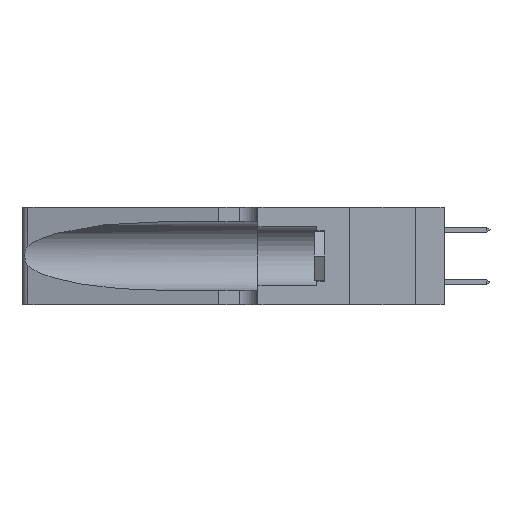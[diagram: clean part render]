
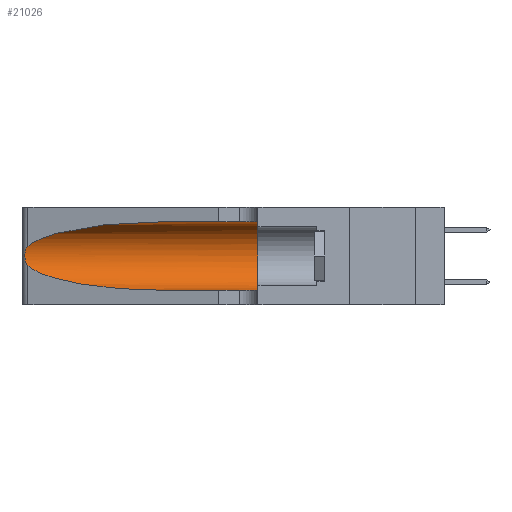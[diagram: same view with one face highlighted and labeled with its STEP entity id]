
A CAD part, left-side view. The second image highlights one B-rep face of the part: STEP entity #21026.
In plain terms, the highlighted cylindrical face has radius 3.308 mm (diameter 6.617 mm), a partial arc.
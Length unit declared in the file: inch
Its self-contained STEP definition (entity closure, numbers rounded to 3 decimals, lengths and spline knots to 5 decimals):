
#993 = CYLINDRICAL_SURFACE ( 'NONE', #23673, 0.13025 ) ;
#1187 = ORIENTED_EDGE ( 'NONE', *, *, #15606, .T. ) ;
#1344 = EDGE_CURVE ( 'NONE', #5291, #2969, #7598, .T. ) ;
#1790 = CARTESIAN_POINT ( 'NONE',  ( 0.1305, 0.35, 0.31525 ) ) ;
#2310 = CARTESIAN_POINT ( 'NONE',  ( 0.25555, 1.22993, 0.14849 ) ) ;
#2969 = VERTEX_POINT ( 'NONE', #16000 ) ;
#3154 = ORIENTED_EDGE ( 'NONE', *, *, #1344, .T. ) ;
#3229 = DIRECTION ( 'NONE',  ( 0., 0., -1. ) ) ;
#3460 = AXIS2_PLACEMENT_3D ( 'NONE', #23264, #11478, #3803 ) ;
#3540 = VERTEX_POINT ( 'NONE', #1790 ) ;
#3803 = DIRECTION ( 'NONE',  ( 0., 0., 1. ) ) ;
#4047 = VERTEX_POINT ( 'NONE', #6953 ) ;
#4234 = CARTESIAN_POINT ( 'NONE',  ( 0.25487, 1.22718, 0.22369 ) ) ;
#4408 = CARTESIAN_POINT ( 'NONE',  ( 0.26017, 1.23833, 0.17102 ) ) ;
#4570 = CARTESIAN_POINT ( 'NONE',  ( 0.1305, 1.61858, 0.05475 ) ) ;
#5130 = VECTOR ( 'NONE', #18428, 39.37008 ) ;
#5291 = VERTEX_POINT ( 'NONE', #11440 ) ;
#6953 = CARTESIAN_POINT ( 'NONE',  ( 0.1305, 0.72297, 0.31525 ) ) ;
#7598 = B_SPLINE_CURVE_WITH_KNOTS ( 'NONE', 3,
 ( #4234, #14229, #23850, #16210, #21959, #12078, #18184, #8489, #4408, #24016, #8404, #12253, #2310, #18264 ),
 .UNSPECIFIED., .F., .F.,
 ( 4, 2, 2, 2, 2, 2, 4 ),
 ( 0., 0.00027, 0.00053, 0.00107, 0.0016, 0.00187, 0.00214 ),
 .UNSPECIFIED. ) ;
#7819 = ORIENTED_EDGE ( 'NONE', *, *, #8131, .F. ) ;
#8131 = EDGE_CURVE ( 'NONE', #4047, #3540, #8203, .T. ) ;
#8194 = EDGE_CURVE ( 'NONE', #2969, #15204, #14914, .T. ) ;
#8203 = LINE ( 'NONE', #20918, #20862 ) ;
#8404 = CARTESIAN_POINT ( 'NONE',  ( 0.25789, 1.23486, 0.15765 ) ) ;
#8489 = CARTESIAN_POINT ( 'NONE',  ( 0.26075, 1.23896, 0.178 ) ) ;
#9005 = DIRECTION ( 'NONE',  ( 0., -1., 0. ) ) ;
#10164 = CARTESIAN_POINT ( 'NONE',  ( 0.25487, 1.22718, 0.14631 ) ) ;
#10472 =( BOUNDED_CURVE ( )  B_SPLINE_CURVE ( 3, ( #18890, #16655, #25178, #21300 ),
 .UNSPECIFIED., .F., .F. ) 
 B_SPLINE_CURVE_WITH_KNOTS ( ( 4, 4 ),
 ( 1.5708, 2.84003 ),
 .UNSPECIFIED. ) 
 CURVE ( )  GEOMETRIC_REPRESENTATION_ITEM ( )  RATIONAL_B_SPLINE_CURVE ( ( 1., 0.87, 0.87, 1. ) ) 
 REPRESENTATION_ITEM ( '' )  );
#11344 = CARTESIAN_POINT ( 'NONE',  ( 0.1305, 0.72297, 0.05475 ) ) ;
#11440 = CARTESIAN_POINT ( 'NONE',  ( 0.25487, 1.22718, 0.22369 ) ) ;
#11478 = DIRECTION ( 'NONE',  ( 0., 1., 0. ) ) ;
#12008 = CARTESIAN_POINT ( 'NONE',  ( 0.1305, 0.35, 0.05475 ) ) ;
#12078 = CARTESIAN_POINT ( 'NONE',  ( 0.26018, 1.23835, 0.19895 ) ) ;
#12253 = CARTESIAN_POINT ( 'NONE',  ( 0.25639, 1.23186, 0.15144 ) ) ;
#13039 = ORIENTED_EDGE ( 'NONE', *, *, #8194, .T. ) ;
#13088 = DIRECTION ( 'NONE',  ( 0., -1., 0. ) ) ;
#13387 = CARTESIAN_POINT ( 'NONE',  ( 0.1305, 0.72297, 0.05475 ) ) ;
#13410 = ORIENTED_EDGE ( 'NONE', *, *, #22148, .F. ) ;
#13567 = CARTESIAN_POINT ( 'NONE',  ( 0.18966, 0.96281, 0.05475 ) ) ;
#14229 = CARTESIAN_POINT ( 'NONE',  ( 0.25555, 1.22994, 0.2215 ) ) ;
#14904 = CARTESIAN_POINT ( 'NONE',  ( 0.1305, 1.61858, 0.185 ) ) ;
#14914 =( BOUNDED_CURVE ( )  B_SPLINE_CURVE ( 3, ( #10164, #18414, #13567, #13387 ),
 .UNSPECIFIED., .F., .T. ) 
 B_SPLINE_CURVE_WITH_KNOTS ( ( 4, 4 ),
 ( 3.44316, 4.71239 ),
 .UNSPECIFIED. ) 
 CURVE ( )  GEOMETRIC_REPRESENTATION_ITEM ( )  RATIONAL_B_SPLINE_CURVE ( ( 1., 0.87, 0.87, 1. ) ) 
 REPRESENTATION_ITEM ( '' )  );
#15204 = VERTEX_POINT ( 'NONE', #11344 ) ;
#15606 = EDGE_CURVE ( 'NONE', #4047, #5291, #10472, .T. ) ;
#15770 = EDGE_LOOP ( 'NONE', ( #1187, #3154, #13039, #19135, #13410, #7819 ) ) ;
#16000 = CARTESIAN_POINT ( 'NONE',  ( 0.25487, 1.22718, 0.14631 ) ) ;
#16210 = CARTESIAN_POINT ( 'NONE',  ( 0.25787, 1.23484, 0.2124 ) ) ;
#16655 = CARTESIAN_POINT ( 'NONE',  ( 0.18966, 0.96281, 0.31525 ) ) ;
#18184 = CARTESIAN_POINT ( 'NONE',  ( 0.26075, 1.23896, 0.19203 ) ) ;
#18264 = CARTESIAN_POINT ( 'NONE',  ( 0.25487, 1.22718, 0.14631 ) ) ;
#18358 = FACE_OUTER_BOUND ( 'NONE', #15770, .T. ) ;
#18414 = CARTESIAN_POINT ( 'NONE',  ( 0.2373, 1.15595, 0.08982 ) ) ;
#18428 = DIRECTION ( 'NONE',  ( 0., -1., 0. ) ) ;
#18890 = CARTESIAN_POINT ( 'NONE',  ( 0.1305, 0.72297, 0.31525 ) ) ;
#19131 = EDGE_CURVE ( 'NONE', #15204, #25509, #25521, .T. ) ;
#19135 = ORIENTED_EDGE ( 'NONE', *, *, #19131, .T. ) ;
#20751 = CIRCLE ( 'NONE', #3460, 0.13025 ) ;
#20862 = VECTOR ( 'NONE', #13088, 39.37008 ) ;
#20918 = CARTESIAN_POINT ( 'NONE',  ( 0.1305, 1.61858, 0.31525 ) ) ;
#21026 = ADVANCED_FACE ( 'NONE', ( #18358 ), #993, .F. ) ;
#21300 = CARTESIAN_POINT ( 'NONE',  ( 0.25487, 1.22718, 0.22369 ) ) ;
#21959 = CARTESIAN_POINT ( 'NONE',  ( 0.25854, 1.2359, 0.20912 ) ) ;
#22148 = EDGE_CURVE ( 'NONE', #3540, #25509, #20751, .T. ) ;
#23264 = CARTESIAN_POINT ( 'NONE',  ( 0.1305, 0.35, 0.185 ) ) ;
#23673 = AXIS2_PLACEMENT_3D ( 'NONE', #14904, #9005, #3229 ) ;
#23850 = CARTESIAN_POINT ( 'NONE',  ( 0.25639, 1.23184, 0.21858 ) ) ;
#24016 = CARTESIAN_POINT ( 'NONE',  ( 0.25856, 1.23593, 0.16098 ) ) ;
#25178 = CARTESIAN_POINT ( 'NONE',  ( 0.2373, 1.15595, 0.28018 ) ) ;
#25509 = VERTEX_POINT ( 'NONE', #12008 ) ;
#25521 = LINE ( 'NONE', #4570, #5130 ) ;
